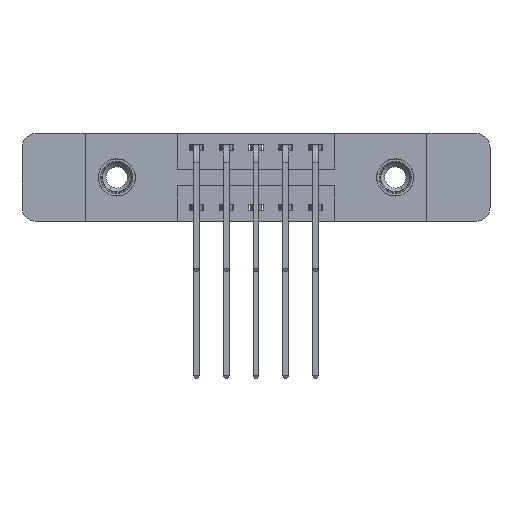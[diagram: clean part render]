
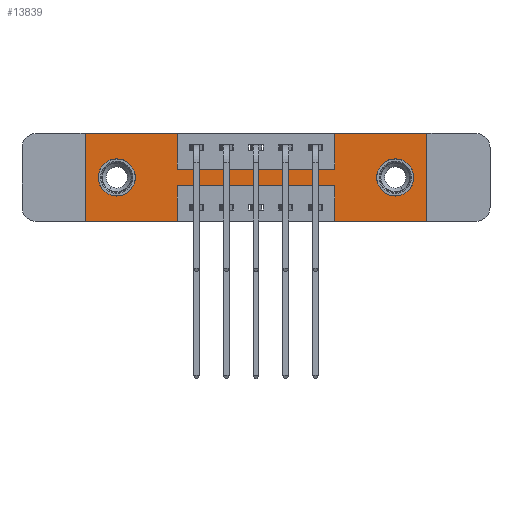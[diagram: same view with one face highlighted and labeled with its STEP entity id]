
A CAD part, front view. The second image highlights one B-rep face of the part: STEP entity #13839.
In plain terms, the highlighted planar face has unit normal (0, -1, 0).
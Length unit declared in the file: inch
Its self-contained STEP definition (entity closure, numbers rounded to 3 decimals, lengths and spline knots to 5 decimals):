
#85 = CARTESIAN_POINT ( 'NONE',  ( 1.435, 0., -0.37 ) ) ;
#320 = DIRECTION ( 'NONE',  ( 0., 0., -1. ) ) ;
#361 = EDGE_CURVE ( 'NONE', #6375, #7342, #6051, .T. ) ;
#424 = VECTOR ( 'NONE', #7130, 39.37008 ) ;
#760 = AXIS2_PLACEMENT_3D ( 'NONE', #8696, #9220, #10093 ) ;
#858 = CARTESIAN_POINT ( 'NONE',  ( 0., 0., 0. ) ) ;
#866 = AXIS2_PLACEMENT_3D ( 'NONE', #5985, #1186, #2308 ) ;
#1145 = VECTOR ( 'NONE', #7071, 39.37008 ) ;
#1172 = CIRCLE ( 'NONE', #760, 0.078 ) ;
#1186 = DIRECTION ( 'NONE',  ( 0., -1., 0. ) ) ;
#1331 = LINE ( 'NONE', #7232, #424 ) ;
#1439 = EDGE_CURVE ( 'NONE', #7342, #6359, #5098, .T. ) ;
#1498 = VERTEX_POINT ( 'NONE', #1886 ) ;
#1504 = CARTESIAN_POINT ( 'NONE',  ( 1.435, 0., 0. ) ) ;
#1543 = VERTEX_POINT ( 'NONE', #10304 ) ;
#1639 = EDGE_LOOP ( 'NONE', ( #2244, #8889 ) ) ;
#1836 = DIRECTION ( 'NONE',  ( 1., 0., 0. ) ) ;
#1886 = CARTESIAN_POINT ( 'NONE',  ( 0.1325, 0., -0.263 ) ) ;
#2018 = LINE ( 'NONE', #11025, #8532 ) ;
#2066 = EDGE_CURVE ( 'NONE', #1498, #3405, #4534, .T. ) ;
#2154 = ORIENTED_EDGE ( 'NONE', *, *, #7048, .F. ) ;
#2207 = CIRCLE ( 'NONE', #12748, 0.078 ) ;
#2244 = ORIENTED_EDGE ( 'NONE', *, *, #5798, .T. ) ;
#2308 = DIRECTION ( 'NONE',  ( 0., 0., -1. ) ) ;
#2337 = CARTESIAN_POINT ( 'NONE',  ( 0., 0., 0. ) ) ;
#2345 = LINE ( 'NONE', #7389, #6638 ) ;
#2615 = LINE ( 'NONE', #2337, #10132 ) ;
#2876 = DIRECTION ( 'NONE',  ( 0., 0., 1. ) ) ;
#3115 = ORIENTED_EDGE ( 'NONE', *, *, #4967, .F. ) ;
#3176 = LINE ( 'NONE', #11024, #12142 ) ;
#3180 = VECTOR ( 'NONE', #12875, 39.37008 ) ;
#3298 = CARTESIAN_POINT ( 'NONE',  ( 1.3025, 0., -0.107 ) ) ;
#3349 = CIRCLE ( 'NONE', #5162, 0.078 ) ;
#3405 = VERTEX_POINT ( 'NONE', #15005 ) ;
#3577 = VECTOR ( 'NONE', #1836, 39.37008 ) ;
#3675 = VECTOR ( 'NONE', #10342, 39.37008 ) ;
#3724 = CARTESIAN_POINT ( 'NONE',  ( 1.3025, 0., -0.263 ) ) ;
#3990 = DIRECTION ( 'NONE',  ( -1., 0., 0. ) ) ;
#4011 = DIRECTION ( 'NONE',  ( 0., 0., -1. ) ) ;
#4058 = CARTESIAN_POINT ( 'NONE',  ( 0.3875, 0., 0. ) ) ;
#4174 = LINE ( 'NONE', #5977, #1145 ) ;
#4511 = ORIENTED_EDGE ( 'NONE', *, *, #1439, .F. ) ;
#4534 = CIRCLE ( 'NONE', #12078, 0.078 ) ;
#4556 = EDGE_CURVE ( 'NONE', #8561, #8502, #10911, .T. ) ;
#4615 = DIRECTION ( 'NONE',  ( -1., 0., 0. ) ) ;
#4725 = CARTESIAN_POINT ( 'NONE',  ( 0., 0., 0. ) ) ;
#4843 = EDGE_CURVE ( 'NONE', #6943, #6375, #13241, .T. ) ;
#4847 = DIRECTION ( 'NONE',  ( 1., 0., 0. ) ) ;
#4967 = EDGE_CURVE ( 'NONE', #1543, #8561, #2615, .T. ) ;
#5060 = DIRECTION ( 'NONE',  ( 0., 0., 1. ) ) ;
#5098 = LINE ( 'NONE', #12200, #3577 ) ;
#5162 = AXIS2_PLACEMENT_3D ( 'NONE', #6540, #12190, #2876 ) ;
#5281 = FACE_BOUND ( 'NONE', #1639, .T. ) ;
#5448 = EDGE_CURVE ( 'NONE', #7218, #10994, #2207, .T. ) ;
#5594 = ORIENTED_EDGE ( 'NONE', *, *, #4556, .F. ) ;
#5670 = VERTEX_POINT ( 'NONE', #5738 ) ;
#5679 = EDGE_LOOP ( 'NONE', ( #14177, #8843, #6399, #7244, #5594, #3115, #2154, #4511, #6650, #10315, #13378, #6303 ) ) ;
#5738 = CARTESIAN_POINT ( 'NONE',  ( 1.0475, 0., -0.37 ) ) ;
#5798 = EDGE_CURVE ( 'NONE', #3405, #1498, #3349, .T. ) ;
#5977 = CARTESIAN_POINT ( 'NONE',  ( 1.0475, 0., 0. ) ) ;
#5985 = CARTESIAN_POINT ( 'NONE',  ( 0., 0., -0.37 ) ) ;
#6051 = LINE ( 'NONE', #9261, #15008 ) ;
#6166 = FACE_BOUND ( 'NONE', #10609, .T. ) ;
#6279 = CARTESIAN_POINT ( 'NONE',  ( 1.0475, 0., -0.15 ) ) ;
#6292 = CARTESIAN_POINT ( 'NONE',  ( 1.3025, 0., -0.185 ) ) ;
#6303 = ORIENTED_EDGE ( 'NONE', *, *, #14571, .F. ) ;
#6359 = VERTEX_POINT ( 'NONE', #6279 ) ;
#6375 = VERTEX_POINT ( 'NONE', #4058 ) ;
#6399 = ORIENTED_EDGE ( 'NONE', *, *, #8884, .F. ) ;
#6463 = DIRECTION ( 'NONE',  ( 0., 1., 0. ) ) ;
#6540 = CARTESIAN_POINT ( 'NONE',  ( 0.1325, 0., -0.185 ) ) ;
#6627 = DIRECTION ( 'NONE',  ( 1., 0., 0. ) ) ;
#6638 = VECTOR ( 'NONE', #4011, 39.37008 ) ;
#6650 = ORIENTED_EDGE ( 'NONE', *, *, #361, .F. ) ;
#6943 = VERTEX_POINT ( 'NONE', #10282 ) ;
#7048 = EDGE_CURVE ( 'NONE', #6359, #1543, #4174, .T. ) ;
#7071 = DIRECTION ( 'NONE',  ( 0., 0., 1. ) ) ;
#7130 = DIRECTION ( 'NONE',  ( -1., 0., 0. ) ) ;
#7218 = VERTEX_POINT ( 'NONE', #3724 ) ;
#7232 = CARTESIAN_POINT ( 'NONE',  ( 0., 0., -0.37 ) ) ;
#7244 = ORIENTED_EDGE ( 'NONE', *, *, #13878, .F. ) ;
#7245 = VERTEX_POINT ( 'NONE', #12652 ) ;
#7342 = VERTEX_POINT ( 'NONE', #14468 ) ;
#7389 = CARTESIAN_POINT ( 'NONE',  ( 0.3875, 0., -0.37 ) ) ;
#7962 = CARTESIAN_POINT ( 'NONE',  ( 0.3875, 0., -0.22 ) ) ;
#8007 = DIRECTION ( 'NONE',  ( 0., 0., -1. ) ) ;
#8164 = ORIENTED_EDGE ( 'NONE', *, *, #5448, .T. ) ;
#8289 = VERTEX_POINT ( 'NONE', #7962 ) ;
#8298 = CARTESIAN_POINT ( 'NONE',  ( 0., 0., -0.37 ) ) ;
#8358 = VECTOR ( 'NONE', #6627, 39.37008 ) ;
#8502 = VERTEX_POINT ( 'NONE', #85 ) ;
#8532 = VECTOR ( 'NONE', #4615, 39.37008 ) ;
#8561 = VERTEX_POINT ( 'NONE', #1504 ) ;
#8696 = CARTESIAN_POINT ( 'NONE',  ( 1.3025, 0., -0.185 ) ) ;
#8843 = ORIENTED_EDGE ( 'NONE', *, *, #11173, .F. ) ;
#8884 = EDGE_CURVE ( 'NONE', #5670, #12857, #9033, .T. ) ;
#8889 = ORIENTED_EDGE ( 'NONE', *, *, #2066, .T. ) ;
#9033 = LINE ( 'NONE', #10431, #3675 ) ;
#9120 = EDGE_CURVE ( 'NONE', #8289, #7245, #2345, .T. ) ;
#9220 = DIRECTION ( 'NONE',  ( 0., 1., 0. ) ) ;
#9261 = CARTESIAN_POINT ( 'NONE',  ( 0.3875, 0., 0. ) ) ;
#9443 = LINE ( 'NONE', #4725, #3180 ) ;
#9749 = CARTESIAN_POINT ( 'NONE',  ( 0.1325, 0., -0.185 ) ) ;
#9971 = VERTEX_POINT ( 'NONE', #8298 ) ;
#10093 = DIRECTION ( 'NONE',  ( 0., 0., -1. ) ) ;
#10126 = ORIENTED_EDGE ( 'NONE', *, *, #12982, .T. ) ;
#10132 = VECTOR ( 'NONE', #4847, 39.37008 ) ;
#10282 = CARTESIAN_POINT ( 'NONE',  ( 0., 0., 0. ) ) ;
#10304 = CARTESIAN_POINT ( 'NONE',  ( 1.0475, 0., 0. ) ) ;
#10315 = ORIENTED_EDGE ( 'NONE', *, *, #4843, .F. ) ;
#10342 = DIRECTION ( 'NONE',  ( 0., 0., 1. ) ) ;
#10431 = CARTESIAN_POINT ( 'NONE',  ( 1.0475, 0., -0.37 ) ) ;
#10502 = CARTESIAN_POINT ( 'NONE',  ( 1.435, 0., 0. ) ) ;
#10609 = EDGE_LOOP ( 'NONE', ( #10126, #8164 ) ) ;
#10911 = LINE ( 'NONE', #10502, #14410 ) ;
#10994 = VERTEX_POINT ( 'NONE', #3298 ) ;
#11024 = CARTESIAN_POINT ( 'NONE',  ( 0.3875, 0., -0.22 ) ) ;
#11025 = CARTESIAN_POINT ( 'NONE',  ( 0., 0., -0.37 ) ) ;
#11173 = EDGE_CURVE ( 'NONE', #12857, #8289, #3176, .T. ) ;
#12002 = DIRECTION ( 'NONE',  ( 0., 1., 0. ) ) ;
#12078 = AXIS2_PLACEMENT_3D ( 'NONE', #9749, #12002, #5060 ) ;
#12142 = VECTOR ( 'NONE', #3990, 39.37008 ) ;
#12190 = DIRECTION ( 'NONE',  ( 0., 1., 0. ) ) ;
#12200 = CARTESIAN_POINT ( 'NONE',  ( 0.3875, 0., -0.15 ) ) ;
#12652 = CARTESIAN_POINT ( 'NONE',  ( 0.3875, 0., -0.37 ) ) ;
#12748 = AXIS2_PLACEMENT_3D ( 'NONE', #6292, #6463, #320 ) ;
#12758 = CARTESIAN_POINT ( 'NONE',  ( 1.0475, 0., -0.22 ) ) ;
#12850 = DIRECTION ( 'NONE',  ( 0., 0., -1. ) ) ;
#12857 = VERTEX_POINT ( 'NONE', #12758 ) ;
#12875 = DIRECTION ( 'NONE',  ( 0., 0., 1. ) ) ;
#12982 = EDGE_CURVE ( 'NONE', #10994, #7218, #1172, .T. ) ;
#13241 = LINE ( 'NONE', #858, #8358 ) ;
#13287 = FACE_OUTER_BOUND ( 'NONE', #5679, .T. ) ;
#13347 = EDGE_CURVE ( 'NONE', #9971, #6943, #9443, .T. ) ;
#13378 = ORIENTED_EDGE ( 'NONE', *, *, #13347, .F. ) ;
#13839 = ADVANCED_FACE ( 'NONE', ( #6166, #5281, #13287 ), #14104, .T. ) ;
#13878 = EDGE_CURVE ( 'NONE', #8502, #5670, #1331, .T. ) ;
#14104 = PLANE ( 'NONE',  #866 ) ;
#14177 = ORIENTED_EDGE ( 'NONE', *, *, #9120, .F. ) ;
#14410 = VECTOR ( 'NONE', #12850, 39.37008 ) ;
#14468 = CARTESIAN_POINT ( 'NONE',  ( 0.3875, 0., -0.15 ) ) ;
#14571 = EDGE_CURVE ( 'NONE', #7245, #9971, #2018, .T. ) ;
#15005 = CARTESIAN_POINT ( 'NONE',  ( 0.1325, 0., -0.107 ) ) ;
#15008 = VECTOR ( 'NONE', #8007, 39.37008 ) ;
